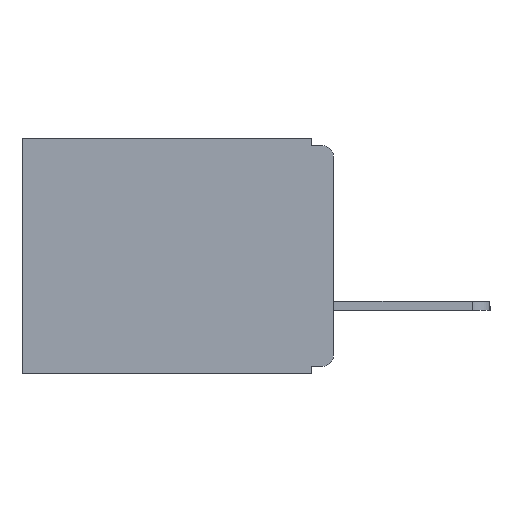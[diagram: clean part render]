
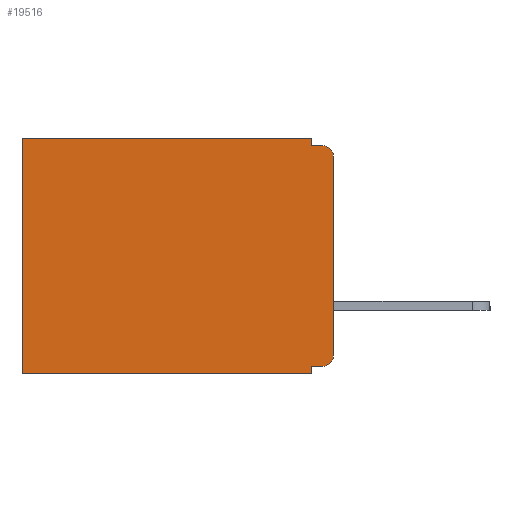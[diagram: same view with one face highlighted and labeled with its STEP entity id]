
A CAD part, left-side view. The second image highlights one B-rep face of the part: STEP entity #19516.
In plain terms, the highlighted planar face has unit normal (-1, 0, 0).
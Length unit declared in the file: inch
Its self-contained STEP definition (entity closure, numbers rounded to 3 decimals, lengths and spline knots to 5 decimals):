
#275 = CARTESIAN_POINT ( 'NONE',  ( 0.3, 0., -0.025 ) ) ;
#782 = EDGE_CURVE ( 'NONE', #33489, #1927, #5173, .T. ) ;
#975 = VECTOR ( 'NONE', #30481, 39.37008 ) ;
#1256 = DIRECTION ( 'NONE',  ( 0., 0., -1. ) ) ;
#1720 = VERTEX_POINT ( 'NONE', #5360 ) ;
#1733 = DIRECTION ( 'NONE',  ( 0., 0., -1. ) ) ;
#1927 = VERTEX_POINT ( 'NONE', #28429 ) ;
#2182 = ORIENTED_EDGE ( 'NONE', *, *, #13891, .F. ) ;
#2316 = CARTESIAN_POINT ( 'NONE',  ( 0.3, 0.031, -0.01 ) ) ;
#2796 = VECTOR ( 'NONE', #33190, 39.37008 ) ;
#2960 = VERTEX_POINT ( 'NONE', #275 ) ;
#3376 = CARTESIAN_POINT ( 'NONE',  ( 0.3, 0., -0.32 ) ) ;
#3461 = EDGE_CURVE ( 'NONE', #4357, #15619, #3971, .T. ) ;
#3573 = DIRECTION ( 'NONE',  ( 0., 1., 0. ) ) ;
#3971 = LINE ( 'NONE', #4814, #16964 ) ;
#4021 = CARTESIAN_POINT ( 'NONE',  ( 0.3, 0.015, -0.025 ) ) ;
#4208 = LINE ( 'NONE', #3376, #10318 ) ;
#4357 = VERTEX_POINT ( 'NONE', #21765 ) ;
#4369 = ORIENTED_EDGE ( 'NONE', *, *, #5508, .F. ) ;
#4814 = CARTESIAN_POINT ( 'NONE',  ( 0.3, 0.031, -0.33 ) ) ;
#5173 = LINE ( 'NONE', #14824, #18147 ) ;
#5322 = ORIENTED_EDGE ( 'NONE', *, *, #3461, .F. ) ;
#5360 = CARTESIAN_POINT ( 'NONE',  ( 0.3, 0.015, -0.01 ) ) ;
#5508 = EDGE_CURVE ( 'NONE', #29179, #4357, #4208, .T. ) ;
#6395 = DIRECTION ( 'NONE',  ( -1., 0., 0. ) ) ;
#6647 = DIRECTION ( 'NONE',  ( 0., 0., -1. ) ) ;
#7921 = FACE_OUTER_BOUND ( 'NONE', #12071, .T. ) ;
#7947 = LINE ( 'NONE', #27921, #975 ) ;
#8072 = VERTEX_POINT ( 'NONE', #21197 ) ;
#8549 = EDGE_CURVE ( 'NONE', #2960, #1720, #8957, .T. ) ;
#8957 = CIRCLE ( 'NONE', #26672, 0.015 ) ;
#9214 = CIRCLE ( 'NONE', #22123, 0.015 ) ;
#9361 = DIRECTION ( 'NONE',  ( 0., 0., -1. ) ) ;
#10318 = VECTOR ( 'NONE', #3573, 39.37008 ) ;
#10698 = AXIS2_PLACEMENT_3D ( 'NONE', #17033, #24849, #9361 ) ;
#10868 = EDGE_CURVE ( 'NONE', #15619, #8072, #15236, .T. ) ;
#11812 = PLANE ( 'NONE',  #10698 ) ;
#12071 = EDGE_LOOP ( 'NONE', ( #26644, #30055, #27304, #2182, #15633, #27750, #33106, #5322, #4369, #24142 ) ) ;
#13891 = EDGE_CURVE ( 'NONE', #33489, #33220, #21618, .T. ) ;
#14824 = CARTESIAN_POINT ( 'NONE',  ( 0.3, 0., 0. ) ) ;
#15049 = CARTESIAN_POINT ( 'NONE',  ( 0.3, 0., -0.01 ) ) ;
#15236 = LINE ( 'NONE', #16697, #28140 ) ;
#15495 = VECTOR ( 'NONE', #1256, 39.37008 ) ;
#15619 = VERTEX_POINT ( 'NONE', #17796 ) ;
#15633 = ORIENTED_EDGE ( 'NONE', *, *, #782, .T. ) ;
#16151 = DIRECTION ( 'NONE',  ( 0., 1., 0. ) ) ;
#16697 = CARTESIAN_POINT ( 'NONE',  ( 0.3, 0., -0.33 ) ) ;
#16837 = CARTESIAN_POINT ( 'NONE',  ( 0.3, 0.031, 0. ) ) ;
#16902 = VECTOR ( 'NONE', #27408, 39.37008 ) ;
#16964 = VECTOR ( 'NONE', #1733, 39.37008 ) ;
#17033 = CARTESIAN_POINT ( 'NONE',  ( 0.3, 0., -0.33 ) ) ;
#17796 = CARTESIAN_POINT ( 'NONE',  ( 0.3, 0.031, -0.33 ) ) ;
#18147 = VECTOR ( 'NONE', #16151, 39.37008 ) ;
#19335 = DIRECTION ( 'NONE',  ( 0., 1., 0. ) ) ;
#19516 = ADVANCED_FACE ( 'NONE', ( #7921 ), #11812, .F. ) ;
#20968 = VERTEX_POINT ( 'NONE', #31056 ) ;
#21197 = CARTESIAN_POINT ( 'NONE',  ( 0.3, 0.437, -0.33 ) ) ;
#21618 = LINE ( 'NONE', #16837, #15495 ) ;
#21765 = CARTESIAN_POINT ( 'NONE',  ( 0.3, 0.031, -0.32 ) ) ;
#21925 = CARTESIAN_POINT ( 'NONE',  ( 0.3, 0.015, -0.305 ) ) ;
#22123 = AXIS2_PLACEMENT_3D ( 'NONE', #21925, #6395, #24516 ) ;
#22189 = DIRECTION ( 'NONE',  ( -1., 0., 0. ) ) ;
#24142 = ORIENTED_EDGE ( 'NONE', *, *, #24808, .T. ) ;
#24516 = DIRECTION ( 'NONE',  ( 0., 0., -1. ) ) ;
#24808 = EDGE_CURVE ( 'NONE', #29179, #20968, #9214, .T. ) ;
#24849 = DIRECTION ( 'NONE',  ( 1., 0., 0. ) ) ;
#24870 = CARTESIAN_POINT ( 'NONE',  ( 0.3, 0.437, -0.33 ) ) ;
#26574 = CARTESIAN_POINT ( 'NONE',  ( 0.3, 0.031, 0. ) ) ;
#26644 = ORIENTED_EDGE ( 'NONE', *, *, #30148, .F. ) ;
#26672 = AXIS2_PLACEMENT_3D ( 'NONE', #4021, #22189, #6647 ) ;
#27304 = ORIENTED_EDGE ( 'NONE', *, *, #33183, .F. ) ;
#27408 = DIRECTION ( 'NONE',  ( 0., 0., -1. ) ) ;
#27750 = ORIENTED_EDGE ( 'NONE', *, *, #29422, .T. ) ;
#27921 = CARTESIAN_POINT ( 'NONE',  ( 0.3, 0., -0.33 ) ) ;
#28140 = VECTOR ( 'NONE', #19335, 39.37008 ) ;
#28429 = CARTESIAN_POINT ( 'NONE',  ( 0.3, 0.437, 0. ) ) ;
#29179 = VERTEX_POINT ( 'NONE', #31459 ) ;
#29422 = EDGE_CURVE ( 'NONE', #1927, #8072, #31392, .T. ) ;
#30055 = ORIENTED_EDGE ( 'NONE', *, *, #8549, .T. ) ;
#30148 = EDGE_CURVE ( 'NONE', #2960, #20968, #7947, .T. ) ;
#30285 = LINE ( 'NONE', #15049, #2796 ) ;
#30481 = DIRECTION ( 'NONE',  ( 0., 0., -1. ) ) ;
#31056 = CARTESIAN_POINT ( 'NONE',  ( 0.3, 0., -0.305 ) ) ;
#31392 = LINE ( 'NONE', #24870, #16902 ) ;
#31459 = CARTESIAN_POINT ( 'NONE',  ( 0.3, 0.015, -0.32 ) ) ;
#33106 = ORIENTED_EDGE ( 'NONE', *, *, #10868, .F. ) ;
#33183 = EDGE_CURVE ( 'NONE', #33220, #1720, #30285, .T. ) ;
#33190 = DIRECTION ( 'NONE',  ( 0., -1., 0. ) ) ;
#33220 = VERTEX_POINT ( 'NONE', #2316 ) ;
#33489 = VERTEX_POINT ( 'NONE', #26574 ) ;
